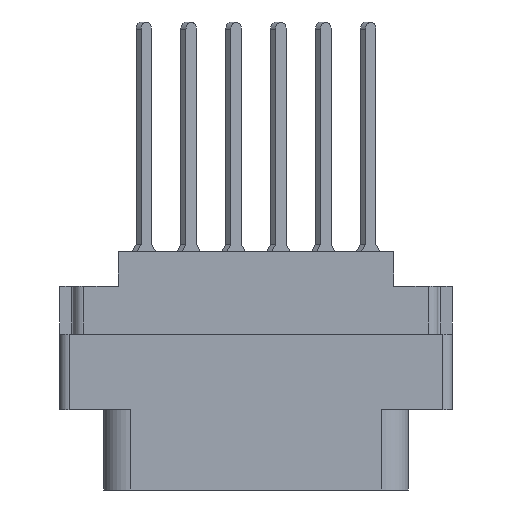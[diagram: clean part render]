
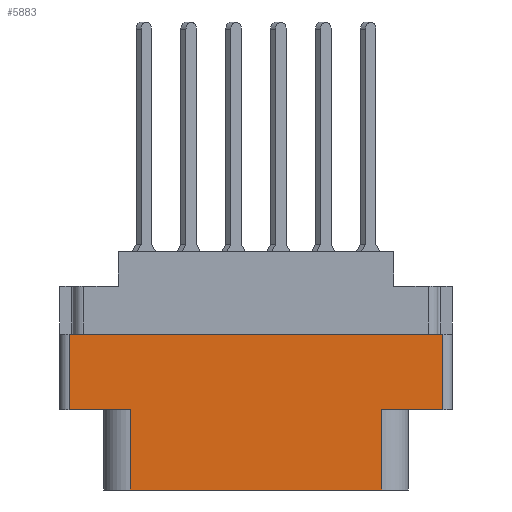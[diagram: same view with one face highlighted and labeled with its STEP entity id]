
A CAD part, front view. The second image highlights one B-rep face of the part: STEP entity #5883.
In plain terms, the highlighted planar face has unit normal (0, -1, 0).
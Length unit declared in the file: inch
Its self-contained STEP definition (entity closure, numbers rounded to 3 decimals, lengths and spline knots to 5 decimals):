
#69 = CARTESIAN_POINT ( 'NONE',  ( 0.42, -0.343, -0.798 ) ) ;
#357 = DIRECTION ( 'NONE',  ( 0., 0., -1. ) ) ;
#369 = CARTESIAN_POINT ( 'NONE',  ( -0.624, -0.343, -0.798 ) ) ;
#794 = DIRECTION ( 'NONE',  ( 0., 0., -1. ) ) ;
#1048 = CARTESIAN_POINT ( 'NONE',  ( 0., -0.343, -0.529 ) ) ;
#1331 = VECTOR ( 'NONE', #357, 39.37008 ) ;
#1637 = LINE ( 'NONE', #6316, #1943 ) ;
#1750 = VERTEX_POINT ( 'NONE', #11235 ) ;
#1943 = VECTOR ( 'NONE', #794, 39.37008 ) ;
#2052 = CARTESIAN_POINT ( 'NONE',  ( -0.656, -0.343, -0.277 ) ) ;
#3209 = VECTOR ( 'NONE', #23718, 39.37008 ) ;
#3668 = VERTEX_POINT ( 'NONE', #9228 ) ;
#4269 = LINE ( 'NONE', #7699, #1331 ) ;
#4740 = ORIENTED_EDGE ( 'NONE', *, *, #8855, .T. ) ;
#4933 = CARTESIAN_POINT ( 'NONE',  ( 0.42, -0.343, -0.529 ) ) ;
#5058 = LINE ( 'NONE', #369, #5344 ) ;
#5344 = VECTOR ( 'NONE', #15136, 39.37008 ) ;
#5590 = LINE ( 'NONE', #17750, #12025 ) ;
#5651 = VERTEX_POINT ( 'NONE', #18753 ) ;
#5659 = VECTOR ( 'NONE', #15950, 39.37008 ) ;
#5883 = ADVANCED_FACE ( 'NONE', ( #21400 ), #23444, .T. ) ;
#6231 = EDGE_CURVE ( 'NONE', #3668, #16860, #5058, .T. ) ;
#6305 = ORIENTED_EDGE ( 'NONE', *, *, #23435, .T. ) ;
#6316 = CARTESIAN_POINT ( 'NONE',  ( 0.42, -0.343, -0.529 ) ) ;
#6372 = DIRECTION ( 'NONE',  ( 0., 0., -1. ) ) ;
#6918 = EDGE_CURVE ( 'NONE', #12199, #11250, #1637, .T. ) ;
#7030 = VERTEX_POINT ( 'NONE', #8138 ) ;
#7276 = EDGE_CURVE ( 'NONE', #16860, #1750, #8865, .T. ) ;
#7355 = CARTESIAN_POINT ( 'NONE',  ( -0.624, -0.343, -0.277 ) ) ;
#7699 = CARTESIAN_POINT ( 'NONE',  ( -0.42, -0.343, -0.529 ) ) ;
#7705 = VECTOR ( 'NONE', #22699, 39.37008 ) ;
#8138 = CARTESIAN_POINT ( 'NONE',  ( -0.42, -0.343, -0.798 ) ) ;
#8176 = LINE ( 'NONE', #21965, #3209 ) ;
#8855 = EDGE_CURVE ( 'NONE', #7030, #11250, #5590, .T. ) ;
#8865 = LINE ( 'NONE', #2052, #7705 ) ;
#9228 = CARTESIAN_POINT ( 'NONE',  ( -0.624, -0.343, -0.529 ) ) ;
#11235 = CARTESIAN_POINT ( 'NONE',  ( 0.624, -0.343, -0.277 ) ) ;
#11250 = VERTEX_POINT ( 'NONE', #69 ) ;
#12025 = VECTOR ( 'NONE', #19660, 39.37008 ) ;
#12199 = VERTEX_POINT ( 'NONE', #4933 ) ;
#12315 = ORIENTED_EDGE ( 'NONE', *, *, #6231, .F. ) ;
#12441 = EDGE_CURVE ( 'NONE', #5651, #7030, #4269, .T. ) ;
#13061 = ORIENTED_EDGE ( 'NONE', *, *, #18787, .F. ) ;
#13741 = ORIENTED_EDGE ( 'NONE', *, *, #7276, .F. ) ;
#13830 = CARTESIAN_POINT ( 'NONE',  ( -0.624, -0.343, -0.798 ) ) ;
#13912 = DIRECTION ( 'NONE',  ( 0., -1., 0. ) ) ;
#13913 = CARTESIAN_POINT ( 'NONE',  ( 0.624, -0.343, -0.798 ) ) ;
#15136 = DIRECTION ( 'NONE',  ( 0., 0., 1. ) ) ;
#15950 = DIRECTION ( 'NONE',  ( 0., 0., 1. ) ) ;
#15992 = DIRECTION ( 'NONE',  ( -1., 0., 0. ) ) ;
#16149 = ORIENTED_EDGE ( 'NONE', *, *, #12441, .T. ) ;
#16492 = LINE ( 'NONE', #13913, #5659 ) ;
#16860 = VERTEX_POINT ( 'NONE', #7355 ) ;
#17750 = CARTESIAN_POINT ( 'NONE',  ( -0.624, -0.343, -0.798 ) ) ;
#18753 = CARTESIAN_POINT ( 'NONE',  ( -0.42, -0.343, -0.529 ) ) ;
#18787 = EDGE_CURVE ( 'NONE', #19414, #12199, #19076, .T. ) ;
#19076 = LINE ( 'NONE', #1048, #22854 ) ;
#19084 = ORIENTED_EDGE ( 'NONE', *, *, #6918, .F. ) ;
#19414 = VERTEX_POINT ( 'NONE', #24015 ) ;
#19660 = DIRECTION ( 'NONE',  ( 1., 0., 0. ) ) ;
#20705 = EDGE_CURVE ( 'NONE', #3668, #5651, #8176, .T. ) ;
#21400 = FACE_OUTER_BOUND ( 'NONE', #24089, .T. ) ;
#21404 = ORIENTED_EDGE ( 'NONE', *, *, #20705, .T. ) ;
#21965 = CARTESIAN_POINT ( 'NONE',  ( 0., -0.343, -0.529 ) ) ;
#22107 = AXIS2_PLACEMENT_3D ( 'NONE', #13830, #13912, #6372 ) ;
#22699 = DIRECTION ( 'NONE',  ( 1., 0., 0. ) ) ;
#22854 = VECTOR ( 'NONE', #15992, 39.37008 ) ;
#23435 = EDGE_CURVE ( 'NONE', #19414, #1750, #16492, .T. ) ;
#23444 = PLANE ( 'NONE',  #22107 ) ;
#23718 = DIRECTION ( 'NONE',  ( 1., 0., 0. ) ) ;
#24015 = CARTESIAN_POINT ( 'NONE',  ( 0.624, -0.343, -0.529 ) ) ;
#24089 = EDGE_LOOP ( 'NONE', ( #16149, #4740, #19084, #13061, #6305, #13741, #12315, #21404 ) ) ;
